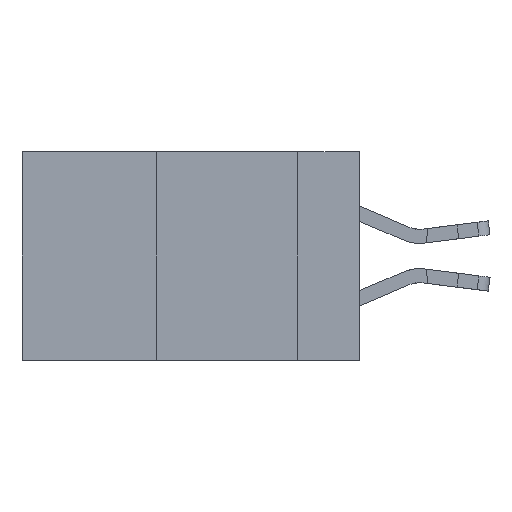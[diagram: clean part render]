
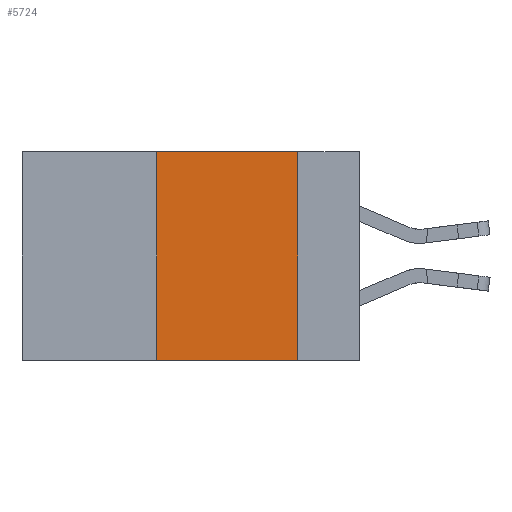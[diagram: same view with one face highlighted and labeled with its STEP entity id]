
A CAD part, left-side view. The second image highlights one B-rep face of the part: STEP entity #5724.
In plain terms, the highlighted planar face has unit normal (-1, 0, 0).
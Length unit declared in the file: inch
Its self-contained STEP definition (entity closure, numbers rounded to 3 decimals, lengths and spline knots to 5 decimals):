
#824 = DIRECTION ( 'NONE',  ( 0., 0., -1. ) ) ;
#1870 = ORIENTED_EDGE ( 'NONE', *, *, #12170, .F. ) ;
#1875 = AXIS2_PLACEMENT_3D ( 'NONE', #14049, #18935, #15120 ) ;
#1949 = DIRECTION ( 'NONE',  ( 0., -1., 0. ) ) ;
#2325 = ORIENTED_EDGE ( 'NONE', *, *, #8686, .T. ) ;
#2697 = VERTEX_POINT ( 'NONE', #10574 ) ;
#3355 = CARTESIAN_POINT ( 'NONE',  ( 0., 0.36, 0. ) ) ;
#3605 = CARTESIAN_POINT ( 'NONE',  ( 0., 0.11, 0. ) ) ;
#4539 = VECTOR ( 'NONE', #1949, 39.37008 ) ;
#5044 = CARTESIAN_POINT ( 'NONE',  ( 0., 0.36, 0. ) ) ;
#5206 = VERTEX_POINT ( 'NONE', #5044 ) ;
#5724 = ADVANCED_FACE ( 'NONE', ( #10686 ), #14068, .F. ) ;
#5996 = CARTESIAN_POINT ( 'NONE',  ( 0., 0.36, -0.37 ) ) ;
#7453 = VECTOR ( 'NONE', #15118, 39.37008 ) ;
#7824 = CARTESIAN_POINT ( 'NONE',  ( 0., 0.6, 0. ) ) ;
#8608 = EDGE_LOOP ( 'NONE', ( #18049, #1870, #11771, #2325 ) ) ;
#8686 = EDGE_CURVE ( 'NONE', #14912, #2697, #14947, .T. ) ;
#8854 = LINE ( 'NONE', #3355, #7453 ) ;
#9160 = EDGE_CURVE ( 'NONE', #9742, #2697, #14477, .T. ) ;
#9742 = VERTEX_POINT ( 'NONE', #3605 ) ;
#10072 = DIRECTION ( 'NONE',  ( 0., -1., 0. ) ) ;
#10574 = CARTESIAN_POINT ( 'NONE',  ( 0., 0.11, -0.37 ) ) ;
#10686 = FACE_OUTER_BOUND ( 'NONE', #8608, .T. ) ;
#11771 = ORIENTED_EDGE ( 'NONE', *, *, #15052, .F. ) ;
#12170 = EDGE_CURVE ( 'NONE', #5206, #9742, #12841, .T. ) ;
#12841 = LINE ( 'NONE', #7824, #4539 ) ;
#14018 = VECTOR ( 'NONE', #824, 39.37008 ) ;
#14049 = CARTESIAN_POINT ( 'NONE',  ( 0., 0.6, 0. ) ) ;
#14068 = PLANE ( 'NONE',  #1875 ) ;
#14477 = LINE ( 'NONE', #15518, #14018 ) ;
#14912 = VERTEX_POINT ( 'NONE', #5996 ) ;
#14947 = LINE ( 'NONE', #17445, #18456 ) ;
#15052 = EDGE_CURVE ( 'NONE', #14912, #5206, #8854, .T. ) ;
#15118 = DIRECTION ( 'NONE',  ( 0., 0., 1. ) ) ;
#15120 = DIRECTION ( 'NONE',  ( 0., 0., -1. ) ) ;
#15518 = CARTESIAN_POINT ( 'NONE',  ( 0., 0.11, 0. ) ) ;
#17445 = CARTESIAN_POINT ( 'NONE',  ( 0., 0.6, -0.37 ) ) ;
#18049 = ORIENTED_EDGE ( 'NONE', *, *, #9160, .F. ) ;
#18456 = VECTOR ( 'NONE', #10072, 39.37008 ) ;
#18935 = DIRECTION ( 'NONE',  ( 1., 0., 0. ) ) ;
